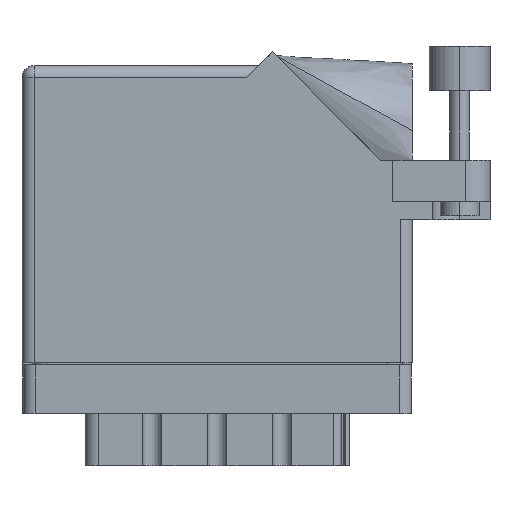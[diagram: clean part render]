
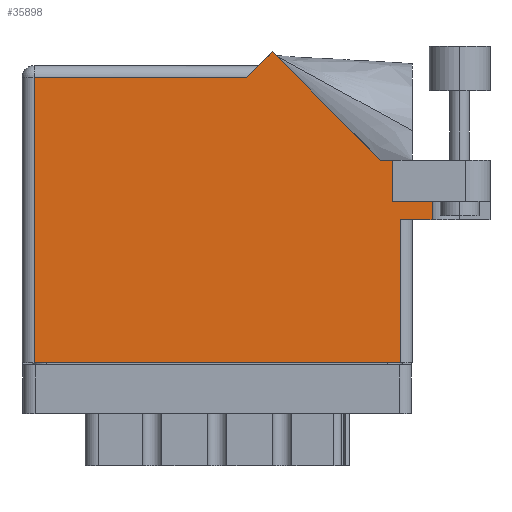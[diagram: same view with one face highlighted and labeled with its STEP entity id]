
A CAD part, front view. The second image highlights one B-rep face of the part: STEP entity #35898.
In plain terms, the highlighted face is planar.
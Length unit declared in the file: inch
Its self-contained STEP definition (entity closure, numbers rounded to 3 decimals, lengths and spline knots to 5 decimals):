
#68 = CARTESIAN_POINT ( 'NONE',  ( 0.062, 1.468, 0. ) ) ;
#604 = VECTOR ( 'NONE', #999, 39.37008 ) ;
#703 = EDGE_LOOP ( 'NONE', ( #20300, #24341, #36926, #20161, #13507, #34309, #29507, #2845, #1330, #34265, #31088 ) ) ;
#734 = CARTESIAN_POINT ( 'NONE',  ( 0., 1.468, 0. ) ) ;
#999 = DIRECTION ( 'NONE',  ( -1., 0., 0. ) ) ;
#1330 = ORIENTED_EDGE ( 'NONE', *, *, #19671, .T. ) ;
#1604 = VERTEX_POINT ( 'NONE', #68 ) ;
#1964 = EDGE_CURVE ( 'NONE', #1604, #36050, #25634, .T. ) ;
#2318 = DIRECTION ( 'NONE',  ( -1., 0., 0. ) ) ;
#2400 = CARTESIAN_POINT ( 'NONE',  ( 1.28771, 1.60071, 0. ) ) ;
#2421 = CARTESIAN_POINT ( 'NONE',  ( 2.1115, 0.737, 0. ) ) ;
#2845 = ORIENTED_EDGE ( 'NONE', *, *, #7194, .T. ) ;
#3468 = DIRECTION ( 'NONE',  ( -0.707, -0.707, 0. ) ) ;
#3600 = VERTEX_POINT ( 'NONE', #2400 ) ;
#4459 = DIRECTION ( 'NONE',  ( 0., -1., 0. ) ) ;
#5134 = VECTOR ( 'NONE', #14948, 39.37008 ) ;
#5581 = DIRECTION ( 'NONE',  ( -1., 0., 0. ) ) ;
#5806 = DIRECTION ( 'NONE',  ( 1., 0., 0. ) ) ;
#6384 = VERTEX_POINT ( 'NONE', #30969 ) ;
#7194 = EDGE_CURVE ( 'NONE', #15406, #3600, #16652, .T. ) ;
#8297 = LINE ( 'NONE', #32386, #5134 ) ;
#8304 = EDGE_CURVE ( 'NONE', #36050, #26045, #29661, .T. ) ;
#9146 = EDGE_CURVE ( 'NONE', #21118, #29816, #35098, .T. ) ;
#9647 = VECTOR ( 'NONE', #10583, 39.37008 ) ;
#10583 = DIRECTION ( 'NONE',  ( 0., 1., 0. ) ) ;
#11541 = CARTESIAN_POINT ( 'NONE',  ( 0., 1.53, 0. ) ) ;
#12629 = EDGE_CURVE ( 'NONE', #26045, #26844, #16218, .T. ) ;
#13188 = CARTESIAN_POINT ( 'NONE',  ( 1.84442, 1.044, 0. ) ) ;
#13333 = VECTOR ( 'NONE', #5806, 39.37008 ) ;
#13507 = ORIENTED_EDGE ( 'NONE', *, *, #9146, .F. ) ;
#14808 = EDGE_CURVE ( 'NONE', #29816, #36430, #8297, .T. ) ;
#14948 = DIRECTION ( 'NONE',  ( 0., -1., 0. ) ) ;
#15256 = EDGE_CURVE ( 'NONE', #21118, #24497, #29538, .T. ) ;
#15406 = VERTEX_POINT ( 'NONE', #28701 ) ;
#15990 = LINE ( 'NONE', #734, #604 ) ;
#16218 = LINE ( 'NONE', #22084, #22994 ) ;
#16652 = LINE ( 'NONE', #13188, #24779 ) ;
#16937 = CARTESIAN_POINT ( 'NONE',  ( 2.01, 0.737, 0. ) ) ;
#17108 = CARTESIAN_POINT ( 'NONE',  ( 1.91, 0.831, 0. ) ) ;
#18646 = DIRECTION ( 'NONE',  ( -0.707, 0.707, 0. ) ) ;
#19631 = CARTESIAN_POINT ( 'NONE',  ( 2.41, 1.044, 0. ) ) ;
#19671 = EDGE_CURVE ( 'NONE', #3600, #6384, #27114, .T. ) ;
#20161 = ORIENTED_EDGE ( 'NONE', *, *, #14808, .F. ) ;
#20300 = ORIENTED_EDGE ( 'NONE', *, *, #8304, .T. ) ;
#20513 = LINE ( 'NONE', #19631, #25065 ) ;
#20779 = CARTESIAN_POINT ( 'NONE',  ( 1.217, 1.53, 0. ) ) ;
#21118 = VERTEX_POINT ( 'NONE', #31787 ) ;
#21195 = VECTOR ( 'NONE', #3468, 39.37008 ) ;
#21977 = VECTOR ( 'NONE', #36124, 39.37008 ) ;
#22084 = CARTESIAN_POINT ( 'NONE',  ( 1.948, 0.737, 0. ) ) ;
#22422 = CARTESIAN_POINT ( 'NONE',  ( 2.1115, 0.831, 0. ) ) ;
#22994 = VECTOR ( 'NONE', #30682, 39.37008 ) ;
#23884 = EDGE_CURVE ( 'NONE', #24497, #15406, #20513, .T. ) ;
#24341 = ORIENTED_EDGE ( 'NONE', *, *, #12629, .T. ) ;
#24409 = VECTOR ( 'NONE', #31343, 39.37008 ) ;
#24497 = VERTEX_POINT ( 'NONE', #33866 ) ;
#24779 = VECTOR ( 'NONE', #18646, 39.37008 ) ;
#25065 = VECTOR ( 'NONE', #2318, 39.37008 ) ;
#25315 = LINE ( 'NONE', #16937, #24409 ) ;
#25537 = CARTESIAN_POINT ( 'NONE',  ( 1.91, 0.831, 0. ) ) ;
#25634 = LINE ( 'NONE', #33540, #36499 ) ;
#26045 = VERTEX_POINT ( 'NONE', #35530 ) ;
#26844 = VERTEX_POINT ( 'NONE', #35302 ) ;
#27114 = LINE ( 'NONE', #20779, #21195 ) ;
#28701 = CARTESIAN_POINT ( 'NONE',  ( 1.84442, 1.044, 0. ) ) ;
#28878 = EDGE_CURVE ( 'NONE', #6384, #1604, #15990, .T. ) ;
#29023 = FACE_OUTER_BOUND ( 'NONE', #703, .T. ) ;
#29507 = ORIENTED_EDGE ( 'NONE', *, *, #23884, .T. ) ;
#29538 = LINE ( 'NONE', #25537, #9647 ) ;
#29661 = LINE ( 'NONE', #33205, #21977 ) ;
#29816 = VERTEX_POINT ( 'NONE', #22422 ) ;
#30682 = DIRECTION ( 'NONE',  ( 0., 1., 0. ) ) ;
#30789 = AXIS2_PLACEMENT_3D ( 'NONE', #11541, #31413, #5581 ) ;
#30969 = CARTESIAN_POINT ( 'NONE',  ( 1.155, 1.468, 0. ) ) ;
#31088 = ORIENTED_EDGE ( 'NONE', *, *, #1964, .T. ) ;
#31343 = DIRECTION ( 'NONE',  ( 1., 0., 0. ) ) ;
#31413 = DIRECTION ( 'NONE',  ( 0., 0., -1. ) ) ;
#31546 = PLANE ( 'NONE',  #30789 ) ;
#31787 = CARTESIAN_POINT ( 'NONE',  ( 1.91, 0.831, 0. ) ) ;
#32386 = CARTESIAN_POINT ( 'NONE',  ( 2.1115, 1.16177, 0. ) ) ;
#33205 = CARTESIAN_POINT ( 'NONE',  ( 0., 0., 0. ) ) ;
#33540 = CARTESIAN_POINT ( 'NONE',  ( 0.062, 0., 0. ) ) ;
#33866 = CARTESIAN_POINT ( 'NONE',  ( 1.91, 1.044, 0. ) ) ;
#34265 = ORIENTED_EDGE ( 'NONE', *, *, #28878, .T. ) ;
#34309 = ORIENTED_EDGE ( 'NONE', *, *, #15256, .T. ) ;
#34816 = CARTESIAN_POINT ( 'NONE',  ( 0.062, 0., 0. ) ) ;
#35098 = LINE ( 'NONE', #17108, #13333 ) ;
#35302 = CARTESIAN_POINT ( 'NONE',  ( 1.948, 0.737, 0. ) ) ;
#35530 = CARTESIAN_POINT ( 'NONE',  ( 1.948, 0., 0. ) ) ;
#35898 = ADVANCED_FACE ( 'NONE', ( #29023 ), #31546, .F. ) ;
#36050 = VERTEX_POINT ( 'NONE', #34816 ) ;
#36124 = DIRECTION ( 'NONE',  ( 1., 0., 0. ) ) ;
#36430 = VERTEX_POINT ( 'NONE', #2421 ) ;
#36499 = VECTOR ( 'NONE', #4459, 39.37008 ) ;
#36926 = ORIENTED_EDGE ( 'NONE', *, *, #36929, .T. ) ;
#36929 = EDGE_CURVE ( 'NONE', #26844, #36430, #25315, .T. ) ;
